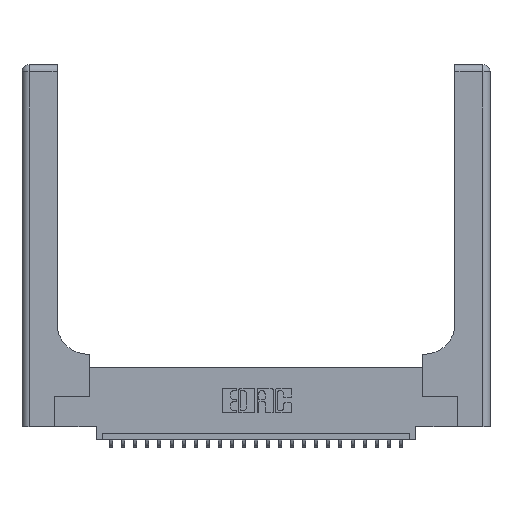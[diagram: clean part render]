
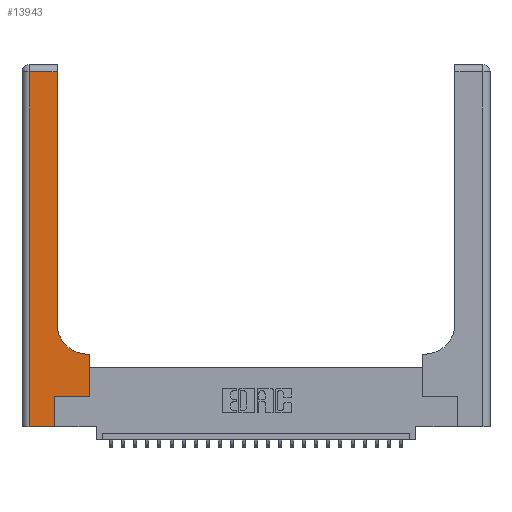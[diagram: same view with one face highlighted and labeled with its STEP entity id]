
A CAD part, top view. The second image highlights one B-rep face of the part: STEP entity #13943.
In plain terms, the highlighted planar face has unit normal (0, 0, 1).
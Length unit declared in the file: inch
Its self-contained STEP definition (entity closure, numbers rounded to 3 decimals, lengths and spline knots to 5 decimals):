
#77 = CARTESIAN_POINT ( 'NONE',  ( 0.2915, 3., 0.37 ) ) ;
#274 = CARTESIAN_POINT ( 'NONE',  ( 0.269, 0.25, 0.37 ) ) ;
#1595 = CARTESIAN_POINT ( 'NONE',  ( 0.269, 0., 0.37 ) ) ;
#1901 = CARTESIAN_POINT ( 'NONE',  ( 0.269, 0.25, 0.37 ) ) ;
#2778 = CARTESIAN_POINT ( 'NONE',  ( 0.06, 2.94, 0.37 ) ) ;
#3441 = EDGE_CURVE ( 'NONE', #15340, #8248, #10002, .T. ) ;
#3747 = CARTESIAN_POINT ( 'NONE',  ( 0., 2.94, 0.37 ) ) ;
#3779 = LINE ( 'NONE', #1595, #13993 ) ;
#3963 = CARTESIAN_POINT ( 'NONE',  ( 0.06, 0., 0.37 ) ) ;
#4246 = EDGE_LOOP ( 'NONE', ( #20755, #17877, #12444, #19812, #19768, #21472, #12262, #26187, #26484 ) ) ;
#4448 = VERTEX_POINT ( 'NONE', #3963 ) ;
#4558 = DIRECTION ( 'NONE',  ( 1., 0., 0. ) ) ;
#5005 = DIRECTION ( 'NONE',  ( -1., 0., 0. ) ) ;
#5602 = VERTEX_POINT ( 'NONE', #1901 ) ;
#6037 = EDGE_CURVE ( 'NONE', #4448, #9741, #21293, .T. ) ;
#6965 = CARTESIAN_POINT ( 'NONE',  ( 0.2915, 0.6, 0.37 ) ) ;
#7059 = PLANE ( 'NONE',  #13005 ) ;
#7486 = DIRECTION ( 'NONE',  ( 1., 0., 0. ) ) ;
#7874 = EDGE_CURVE ( 'NONE', #16855, #10018, #9050, .T. ) ;
#8248 = VERTEX_POINT ( 'NONE', #9912 ) ;
#8360 = CARTESIAN_POINT ( 'NONE',  ( 0.06, 3., 0.37 ) ) ;
#9050 = LINE ( 'NONE', #3747, #24692 ) ;
#9518 = VECTOR ( 'NONE', #5005, 39.37008 ) ;
#9668 = EDGE_CURVE ( 'NONE', #5602, #23718, #10569, .T. ) ;
#9741 = VERTEX_POINT ( 'NONE', #10164 ) ;
#9912 = CARTESIAN_POINT ( 'NONE',  ( 0.2915, 0.85, 0.37 ) ) ;
#10002 = CIRCLE ( 'NONE', #11852, 0.25 ) ;
#10018 = VERTEX_POINT ( 'NONE', #2778 ) ;
#10164 = CARTESIAN_POINT ( 'NONE',  ( 0.269, 0., 0.37 ) ) ;
#10569 = LINE ( 'NONE', #274, #19825 ) ;
#10734 = DIRECTION ( 'NONE',  ( 0., 0., -1. ) ) ;
#11576 = CARTESIAN_POINT ( 'NONE',  ( 0.2915, 2.94, 0.37 ) ) ;
#11852 = AXIS2_PLACEMENT_3D ( 'NONE', #17206, #10734, #4558 ) ;
#12262 = ORIENTED_EDGE ( 'NONE', *, *, #24461, .T. ) ;
#12444 = ORIENTED_EDGE ( 'NONE', *, *, #23704, .T. ) ;
#13005 = AXIS2_PLACEMENT_3D ( 'NONE', #17199, #21346, #23649 ) ;
#13852 = VECTOR ( 'NONE', #16688, 39.37008 ) ;
#13934 = EDGE_CURVE ( 'NONE', #23077, #15340, #24519, .T. ) ;
#13943 = ADVANCED_FACE ( 'NONE', ( #18487 ), #7059, .F. ) ;
#13993 = VECTOR ( 'NONE', #19963, 39.37008 ) ;
#14036 = VECTOR ( 'NONE', #22047, 39.37008 ) ;
#14779 = DIRECTION ( 'NONE',  ( 1., 0., 0. ) ) ;
#15340 = VERTEX_POINT ( 'NONE', #24270 ) ;
#15847 = CARTESIAN_POINT ( 'NONE',  ( 0.5585, 0.25, 0.37 ) ) ;
#16633 = LINE ( 'NONE', #15847, #14036 ) ;
#16688 = DIRECTION ( 'NONE',  ( 0., -1., 0. ) ) ;
#16855 = VERTEX_POINT ( 'NONE', #11576 ) ;
#17199 = CARTESIAN_POINT ( 'NONE',  ( 0., 3., 0.37 ) ) ;
#17206 = CARTESIAN_POINT ( 'NONE',  ( 0.5415, 0.85, 0.37 ) ) ;
#17236 = CARTESIAN_POINT ( 'NONE',  ( 0.5585, 0.25, 0.37 ) ) ;
#17651 = EDGE_CURVE ( 'NONE', #8248, #16855, #23103, .T. ) ;
#17871 = CARTESIAN_POINT ( 'NONE',  ( 0., 0., 0.37 ) ) ;
#17877 = ORIENTED_EDGE ( 'NONE', *, *, #7874, .T. ) ;
#18034 = LINE ( 'NONE', #8360, #13852 ) ;
#18047 = DIRECTION ( 'NONE',  ( -1., 0., 0. ) ) ;
#18487 = FACE_OUTER_BOUND ( 'NONE', #4246, .T. ) ;
#19589 = VECTOR ( 'NONE', #23056, 39.37008 ) ;
#19768 = ORIENTED_EDGE ( 'NONE', *, *, #26468, .T. ) ;
#19812 = ORIENTED_EDGE ( 'NONE', *, *, #6037, .T. ) ;
#19825 = VECTOR ( 'NONE', #14779, 39.37008 ) ;
#19963 = DIRECTION ( 'NONE',  ( 0., 1., 0. ) ) ;
#20176 = CARTESIAN_POINT ( 'NONE',  ( 0.5585, 0.6, 0.37 ) ) ;
#20755 = ORIENTED_EDGE ( 'NONE', *, *, #17651, .T. ) ;
#21293 = LINE ( 'NONE', #17871, #22865 ) ;
#21346 = DIRECTION ( 'NONE',  ( 0., 0., -1. ) ) ;
#21472 = ORIENTED_EDGE ( 'NONE', *, *, #9668, .T. ) ;
#22047 = DIRECTION ( 'NONE',  ( 0., 1., 0. ) ) ;
#22865 = VECTOR ( 'NONE', #7486, 39.37008 ) ;
#23056 = DIRECTION ( 'NONE',  ( 0., 1., 0. ) ) ;
#23077 = VERTEX_POINT ( 'NONE', #20176 ) ;
#23103 = LINE ( 'NONE', #77, #19589 ) ;
#23649 = DIRECTION ( 'NONE',  ( -1., 0., 0. ) ) ;
#23704 = EDGE_CURVE ( 'NONE', #10018, #4448, #18034, .T. ) ;
#23718 = VERTEX_POINT ( 'NONE', #17236 ) ;
#24270 = CARTESIAN_POINT ( 'NONE',  ( 0.5415, 0.6, 0.37 ) ) ;
#24461 = EDGE_CURVE ( 'NONE', #23718, #23077, #16633, .T. ) ;
#24519 = LINE ( 'NONE', #6965, #9518 ) ;
#24692 = VECTOR ( 'NONE', #18047, 39.37008 ) ;
#26187 = ORIENTED_EDGE ( 'NONE', *, *, #13934, .T. ) ;
#26468 = EDGE_CURVE ( 'NONE', #9741, #5602, #3779, .T. ) ;
#26484 = ORIENTED_EDGE ( 'NONE', *, *, #3441, .T. ) ;
